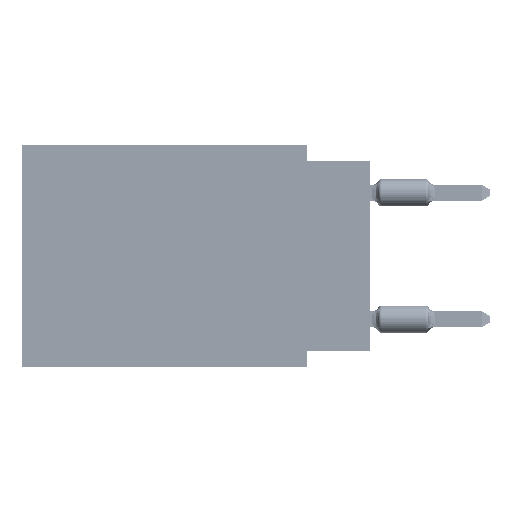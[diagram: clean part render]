
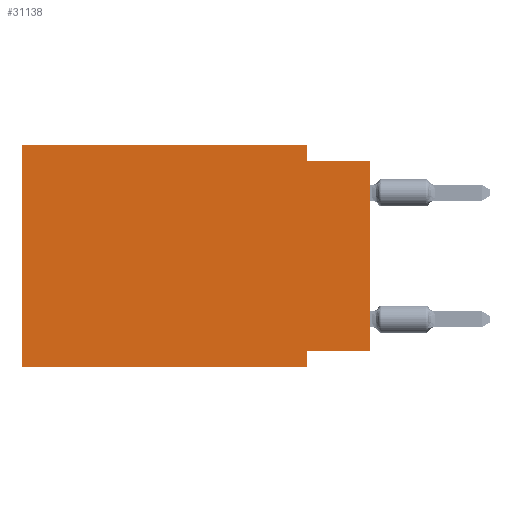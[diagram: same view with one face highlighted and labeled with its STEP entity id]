
A CAD part, left-side view. The second image highlights one B-rep face of the part: STEP entity #31138.
In plain terms, the highlighted planar face has unit normal (-1, 0, 0).
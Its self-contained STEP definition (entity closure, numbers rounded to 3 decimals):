
#2381 = DIRECTION ( 'NONE',  ( 0., 0., 1. ) ) ;
#2827 = ORIENTED_EDGE ( 'NONE', *, *, #47802, .F. ) ;
#3504 = LINE ( 'NONE', #66191, #9638 ) ;
#3507 = FACE_OUTER_BOUND ( 'NONE', #30530, .T. ) ;
#5763 = CARTESIAN_POINT ( 'NONE',  ( 0., 13.97, 0. ) ) ;
#6453 = VERTEX_POINT ( 'NONE', #53799 ) ;
#8715 = VERTEX_POINT ( 'NONE', #13250 ) ;
#9027 = VECTOR ( 'NONE', #15435, 1000. ) ;
#9638 = VECTOR ( 'NONE', #2381, 1000. ) ;
#10091 = VECTOR ( 'NONE', #30359, 1000. ) ;
#10192 = LINE ( 'NONE', #66563, #9027 ) ;
#13250 = CARTESIAN_POINT ( 'NONE',  ( 0., 2.54, 0. ) ) ;
#13874 = DIRECTION ( 'NONE',  ( 0., -1., 0. ) ) ;
#14795 = VERTEX_POINT ( 'NONE', #71073 ) ;
#15435 = DIRECTION ( 'NONE',  ( 0., -1., 0. ) ) ;
#16081 = CARTESIAN_POINT ( 'NONE',  ( 0., 13.97, 0. ) ) ;
#18492 = LINE ( 'NONE', #34893, #68669 ) ;
#20302 = DIRECTION ( 'NONE',  ( 1., 0., 0. ) ) ;
#20564 = ORIENTED_EDGE ( 'NONE', *, *, #27536, .T. ) ;
#22541 = ORIENTED_EDGE ( 'NONE', *, *, #60148, .F. ) ;
#25623 = VERTEX_POINT ( 'NONE', #69600 ) ;
#25975 = DIRECTION ( 'NONE',  ( 0., 0., -1. ) ) ;
#26693 = EDGE_CURVE ( 'NONE', #6453, #70458, #31564, .T. ) ;
#27242 = ORIENTED_EDGE ( 'NONE', *, *, #37493, .T. ) ;
#27536 = EDGE_CURVE ( 'NONE', #59782, #70458, #42223, .T. ) ;
#30359 = DIRECTION ( 'NONE',  ( 0., 0., 1. ) ) ;
#30530 = EDGE_LOOP ( 'NONE', ( #27242, #22541, #2827, #48708, #49023, #20564, #34749, #58157 ) ) ;
#31079 = CARTESIAN_POINT ( 'NONE',  ( 0., 0., -0.635 ) ) ;
#31138 = ADVANCED_FACE ( 'NONE', ( #3507 ), #71426, .F. ) ;
#31564 = LINE ( 'NONE', #65528, #60998 ) ;
#32020 = VECTOR ( 'NONE', #41265, 1000. ) ;
#34749 = ORIENTED_EDGE ( 'NONE', *, *, #26693, .F. ) ;
#34893 = CARTESIAN_POINT ( 'NONE',  ( 0., 2.54, 0. ) ) ;
#35883 = LINE ( 'NONE', #58654, #36249 ) ;
#36249 = VECTOR ( 'NONE', #40772, 1000. ) ;
#37493 = EDGE_CURVE ( 'NONE', #58155, #14795, #3504, .T. ) ;
#37553 = AXIS2_PLACEMENT_3D ( 'NONE', #16081, #20302, #43047 ) ;
#37855 = CARTESIAN_POINT ( 'NONE',  ( 0., 2.54, -8.89 ) ) ;
#40772 = DIRECTION ( 'NONE',  ( 0., 1., 0. ) ) ;
#41265 = DIRECTION ( 'NONE',  ( 0., -1., 0. ) ) ;
#42223 = LINE ( 'NONE', #64256, #64622 ) ;
#43014 = LINE ( 'NONE', #31079, #32020 ) ;
#43047 = DIRECTION ( 'NONE',  ( 0., 0., -1. ) ) ;
#43486 = EDGE_CURVE ( 'NONE', #25623, #8715, #10192, .T. ) ;
#43648 = CARTESIAN_POINT ( 'NONE',  ( 0., 0., -8.255 ) ) ;
#46031 = EDGE_CURVE ( 'NONE', #58155, #6453, #35883, .T. ) ;
#47802 = EDGE_CURVE ( 'NONE', #8715, #54048, #18492, .T. ) ;
#48708 = ORIENTED_EDGE ( 'NONE', *, *, #43486, .F. ) ;
#49023 = ORIENTED_EDGE ( 'NONE', *, *, #52998, .F. ) ;
#52998 = EDGE_CURVE ( 'NONE', #59782, #25623, #68073, .T. ) ;
#53799 = CARTESIAN_POINT ( 'NONE',  ( 0., 2.54, -8.255 ) ) ;
#54048 = VERTEX_POINT ( 'NONE', #71009 ) ;
#58155 = VERTEX_POINT ( 'NONE', #43648 ) ;
#58157 = ORIENTED_EDGE ( 'NONE', *, *, #46031, .F. ) ;
#58654 = CARTESIAN_POINT ( 'NONE',  ( 0., 0., -8.255 ) ) ;
#59782 = VERTEX_POINT ( 'NONE', #70826 ) ;
#60148 = EDGE_CURVE ( 'NONE', #54048, #14795, #43014, .T. ) ;
#60998 = VECTOR ( 'NONE', #25975, 1000. ) ;
#63636 = DIRECTION ( 'NONE',  ( 0., 0., -1. ) ) ;
#64256 = CARTESIAN_POINT ( 'NONE',  ( 0., 13.97, -8.89 ) ) ;
#64622 = VECTOR ( 'NONE', #13874, 1000. ) ;
#65528 = CARTESIAN_POINT ( 'NONE',  ( 0., 2.54, -8.89 ) ) ;
#66191 = CARTESIAN_POINT ( 'NONE',  ( 0., 0., 0. ) ) ;
#66563 = CARTESIAN_POINT ( 'NONE',  ( 0., 13.97, 0. ) ) ;
#68073 = LINE ( 'NONE', #5763, #10091 ) ;
#68669 = VECTOR ( 'NONE', #63636, 1000. ) ;
#69600 = CARTESIAN_POINT ( 'NONE',  ( 0., 13.97, 0. ) ) ;
#70458 = VERTEX_POINT ( 'NONE', #37855 ) ;
#70826 = CARTESIAN_POINT ( 'NONE',  ( 0., 13.97, -8.89 ) ) ;
#71009 = CARTESIAN_POINT ( 'NONE',  ( 0., 2.54, -0.635 ) ) ;
#71073 = CARTESIAN_POINT ( 'NONE',  ( 0., 0., -0.635 ) ) ;
#71426 = PLANE ( 'NONE',  #37553 ) ;
